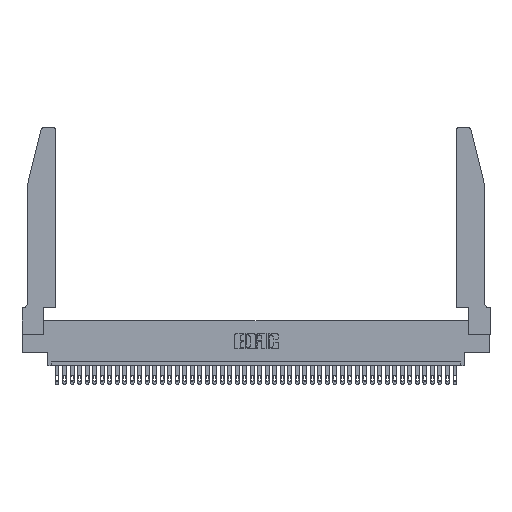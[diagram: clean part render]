
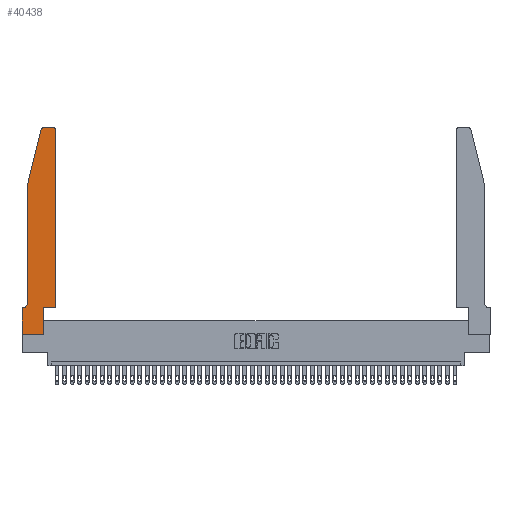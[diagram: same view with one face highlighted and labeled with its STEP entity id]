
A CAD part, top view. The second image highlights one B-rep face of the part: STEP entity #40438.
In plain terms, the highlighted planar face has unit normal (0, 0, 1).
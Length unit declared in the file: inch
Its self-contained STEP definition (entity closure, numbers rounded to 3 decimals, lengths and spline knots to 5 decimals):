
#578 = EDGE_CURVE ( 'NONE', #17467, #13738, #10854, .T. ) ;
#764 = CARTESIAN_POINT ( 'NONE',  ( 0.0755, 0.42, 0.37 ) ) ;
#766 = DIRECTION ( 'NONE',  ( -0.239, -0.971, 0. ) ) ;
#873 = VECTOR ( 'NONE', #23694, 39.37008 ) ;
#2639 = EDGE_CURVE ( 'NONE', #34064, #32188, #23398, .T. ) ;
#3765 = VERTEX_POINT ( 'NONE', #20030 ) ;
#3775 = EDGE_CURVE ( 'NONE', #13483, #17467, #9019, .T. ) ;
#4197 = VERTEX_POINT ( 'NONE', #7678 ) ;
#4663 = CIRCLE ( 'NONE', #30208, 0.03 ) ;
#5368 = VECTOR ( 'NONE', #26877, 39.37008 ) ;
#5617 = DIRECTION ( 'NONE',  ( -1., 0., 0. ) ) ;
#5829 = DIRECTION ( 'NONE',  ( 0., -1., 0. ) ) ;
#5846 = CARTESIAN_POINT ( 'NONE',  ( 0.0755, 2., 0.37 ) ) ;
#5989 = DIRECTION ( 'NONE',  ( 1., 0., 0. ) ) ;
#6912 = VECTOR ( 'NONE', #10256, 39.37008 ) ;
#7328 = CARTESIAN_POINT ( 'NONE',  ( 0., 0.35, 0.37 ) ) ;
#7678 = CARTESIAN_POINT ( 'NONE',  ( 0., 0.35, 0.37 ) ) ;
#7821 = LINE ( 'NONE', #37424, #16313 ) ;
#8003 = CARTESIAN_POINT ( 'NONE',  ( 0.284, 2.72, 0.37 ) ) ;
#8309 = ORIENTED_EDGE ( 'NONE', *, *, #15282, .T. ) ;
#9019 = LINE ( 'NONE', #36862, #6912 ) ;
#9796 = VERTEX_POINT ( 'NONE', #15593 ) ;
#9970 = LINE ( 'NONE', #14064, #873 ) ;
#10150 = ORIENTED_EDGE ( 'NONE', *, *, #39425, .T. ) ;
#10256 = DIRECTION ( 'NONE',  ( 0., 1., 0. ) ) ;
#10854 = LINE ( 'NONE', #19262, #14032 ) ;
#10959 = LINE ( 'NONE', #19024, #21533 ) ;
#11385 = DIRECTION ( 'NONE',  ( 1., 0., 0. ) ) ;
#11980 = DIRECTION ( 'NONE',  ( 0., 0., 1. ) ) ;
#12606 = ORIENTED_EDGE ( 'NONE', *, *, #21763, .T. ) ;
#13059 = EDGE_CURVE ( 'NONE', #34968, #9796, #42901, .T. ) ;
#13483 = VERTEX_POINT ( 'NONE', #40378 ) ;
#13738 = VERTEX_POINT ( 'NONE', #42097 ) ;
#14032 = VECTOR ( 'NONE', #5989, 39.37008 ) ;
#14064 = CARTESIAN_POINT ( 'NONE',  ( 0.0755, 0.35, 0.37 ) ) ;
#14175 = DIRECTION ( 'NONE',  ( 0., 1., 0. ) ) ;
#14251 = EDGE_CURVE ( 'NONE', #9796, #34064, #4663, .T. ) ;
#14307 = EDGE_CURVE ( 'NONE', #33156, #34968, #21600, .T. ) ;
#14519 = EDGE_CURVE ( 'NONE', #13738, #33156, #7821, .T. ) ;
#14984 = CARTESIAN_POINT ( 'NONE',  ( 0.25487, 2.72718, 0.37 ) ) ;
#15282 = EDGE_CURVE ( 'NONE', #32188, #17411, #15706, .T. ) ;
#15593 = CARTESIAN_POINT ( 'NONE',  ( 0.284, 2.75, 0.37 ) ) ;
#15706 = LINE ( 'NONE', #19259, #17828 ) ;
#15780 = DIRECTION ( 'NONE',  ( 0., 0., -1. ) ) ;
#16313 = VECTOR ( 'NONE', #14175, 39.37008 ) ;
#17411 = VERTEX_POINT ( 'NONE', #764 ) ;
#17467 = VERTEX_POINT ( 'NONE', #34717 ) ;
#17828 = VECTOR ( 'NONE', #5829, 39.37008 ) ;
#18362 = ORIENTED_EDGE ( 'NONE', *, *, #14251, .T. ) ;
#18784 = VECTOR ( 'NONE', #24852, 39.37008 ) ;
#19024 = CARTESIAN_POINT ( 'NONE',  ( 0., 0., 0.37 ) ) ;
#19158 = VECTOR ( 'NONE', #766, 39.37008 ) ;
#19175 = DIRECTION ( 'NONE',  ( 0., -1., 0. ) ) ;
#19259 = CARTESIAN_POINT ( 'NONE',  ( 0.0755, 2., 0.37 ) ) ;
#19262 = CARTESIAN_POINT ( 'NONE',  ( 0.4505, 0.35, 0.37 ) ) ;
#19793 = CARTESIAN_POINT ( 'NONE',  ( 0.2605, 2.75, 0.37 ) ) ;
#20030 = CARTESIAN_POINT ( 'NONE',  ( 0.0055, 0.35, 0.37 ) ) ;
#20414 = ORIENTED_EDGE ( 'NONE', *, *, #14519, .T. ) ;
#20597 = ORIENTED_EDGE ( 'NONE', *, *, #14307, .T. ) ;
#21533 = VECTOR ( 'NONE', #19175, 39.37008 ) ;
#21600 = CIRCLE ( 'NONE', #42363, 0.03 ) ;
#21736 = DIRECTION ( 'NONE',  ( 0., 0., 1. ) ) ;
#21763 = EDGE_CURVE ( 'NONE', #3765, #4197, #9970, .T. ) ;
#23398 = LINE ( 'NONE', #35519, #19158 ) ;
#23694 = DIRECTION ( 'NONE',  ( -1., 0., 0. ) ) ;
#24160 = PLANE ( 'NONE',  #38392 ) ;
#24733 = DIRECTION ( 'NONE',  ( 1., 0., 0. ) ) ;
#24852 = DIRECTION ( 'NONE',  ( 1., 0., 0. ) ) ;
#25591 = CARTESIAN_POINT ( 'NONE',  ( 0.4205, 2.72, 0.37 ) ) ;
#25732 = CARTESIAN_POINT ( 'NONE',  ( 0., 0., 0.37 ) ) ;
#25984 = CARTESIAN_POINT ( 'NONE',  ( 0.0055, 0.42, 0.37 ) ) ;
#26595 = ORIENTED_EDGE ( 'NONE', *, *, #2639, .T. ) ;
#26770 = CARTESIAN_POINT ( 'NONE',  ( 0.4205, 2.75, 0.37 ) ) ;
#26877 = DIRECTION ( 'NONE',  ( -1., 0., 0. ) ) ;
#28260 = EDGE_CURVE ( 'NONE', #17411, #3765, #38016, .T. ) ;
#28478 = EDGE_LOOP ( 'NONE', ( #32777, #18362, #26595, #8309, #38076, #12606, #30470, #10150, #31593, #30660, #20414, #20597 ) ) ;
#30208 = AXIS2_PLACEMENT_3D ( 'NONE', #8003, #21736, #11385 ) ;
#30470 = ORIENTED_EDGE ( 'NONE', *, *, #33594, .T. ) ;
#30660 = ORIENTED_EDGE ( 'NONE', *, *, #578, .T. ) ;
#30701 = CARTESIAN_POINT ( 'NONE',  ( 0.4505, 2.72, 0.37 ) ) ;
#31088 = DIRECTION ( 'NONE',  ( 0., 0., 1. ) ) ;
#31593 = ORIENTED_EDGE ( 'NONE', *, *, #3775, .T. ) ;
#31835 = AXIS2_PLACEMENT_3D ( 'NONE', #25984, #15780, #5617 ) ;
#32188 = VERTEX_POINT ( 'NONE', #5846 ) ;
#32777 = ORIENTED_EDGE ( 'NONE', *, *, #13059, .T. ) ;
#33156 = VERTEX_POINT ( 'NONE', #30701 ) ;
#33594 = EDGE_CURVE ( 'NONE', #4197, #36572, #10959, .T. ) ;
#33909 = CARTESIAN_POINT ( 'NONE',  ( 0., 0., 0.37 ) ) ;
#34064 = VERTEX_POINT ( 'NONE', #14984 ) ;
#34549 = FACE_OUTER_BOUND ( 'NONE', #28478, .T. ) ;
#34717 = CARTESIAN_POINT ( 'NONE',  ( 0.2865, 0.35, 0.37 ) ) ;
#34968 = VERTEX_POINT ( 'NONE', #26770 ) ;
#35519 = CARTESIAN_POINT ( 'NONE',  ( 0.0755, 2., 0.37 ) ) ;
#36572 = VERTEX_POINT ( 'NONE', #25732 ) ;
#36862 = CARTESIAN_POINT ( 'NONE',  ( 0.2865, 0.35, 0.37 ) ) ;
#37424 = CARTESIAN_POINT ( 'NONE',  ( 0.4505, 0.35, 0.37 ) ) ;
#38016 = CIRCLE ( 'NONE', #31835, 0.07 ) ;
#38076 = ORIENTED_EDGE ( 'NONE', *, *, #28260, .T. ) ;
#38392 = AXIS2_PLACEMENT_3D ( 'NONE', #7328, #31088, #24733 ) ;
#38747 = DIRECTION ( 'NONE',  ( 1., 0., 0. ) ) ;
#39425 = EDGE_CURVE ( 'NONE', #36572, #13483, #43130, .T. ) ;
#40378 = CARTESIAN_POINT ( 'NONE',  ( 0.2865, 0., 0.37 ) ) ;
#40438 = ADVANCED_FACE ( 'NONE', ( #34549 ), #24160, .T. ) ;
#42097 = CARTESIAN_POINT ( 'NONE',  ( 0.4505, 0.35, 0.37 ) ) ;
#42363 = AXIS2_PLACEMENT_3D ( 'NONE', #25591, #11980, #38747 ) ;
#42901 = LINE ( 'NONE', #19793, #5368 ) ;
#43130 = LINE ( 'NONE', #33909, #18784 ) ;
